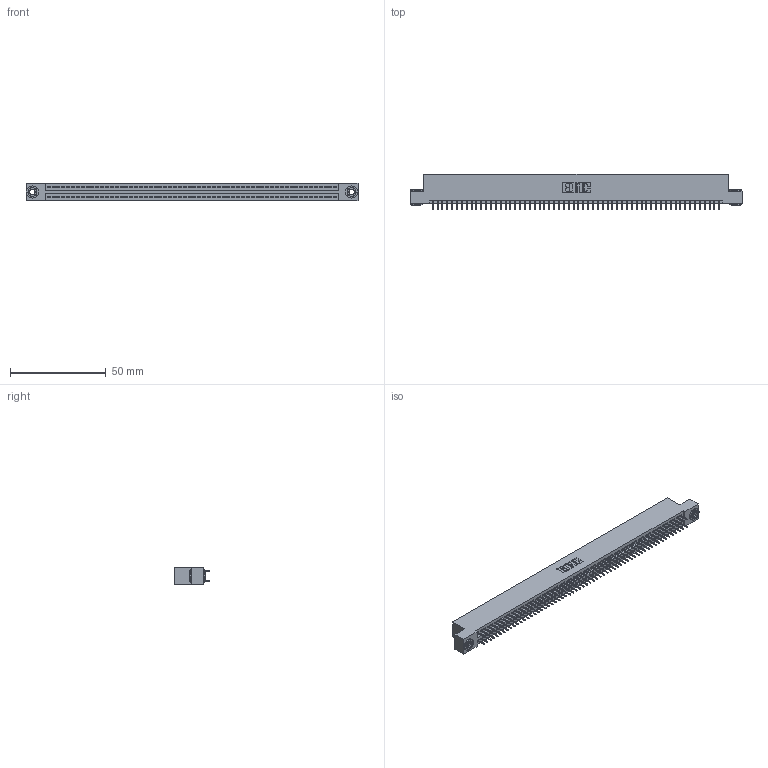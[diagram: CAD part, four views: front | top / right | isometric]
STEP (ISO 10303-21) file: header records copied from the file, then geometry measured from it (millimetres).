
FILE_DESCRIPTION (( 'STEP AP203' ), '1' );
FILE_NAME ('845-120-525-203.STEP', '2020-09-24T09:25:24', ( '' ), ( '' ), 'SwSTEP 2.0', 'SolidWorks 2020', '' );
FILE_SCHEMA (( 'CONFIG_CONTROL_DESIGN' ));
Length unit declared in the file: inch
Products named in the file (4): 345-250-002_345-250-002-102; 845-120-525-203; 345-292-001_345-293-125; 845 Part_Flush Mounting Lugs - 0.156 Dia-TH
Assembly tree (123 placements, depth 2):
  845-120-525-203
    845 Part_Flush Mounting Lugs - 0.156 Dia-TH
    345-292-001_345-293-125  x120
    345-250-002_345-250-002-102  x2
Bounding box: 173.61 x 18.72 x 9.4 mm (x, y, z)
Volume: 16853.5 mm3; surface area: 24870.6 mm2
Topology: 123 solids, 123 shells, 6644 faces, 18777 edges, 12034 vertices
Faces by surface type: plane 4770, cylinder 1866, cone 8
Entity records: 45378 total; most frequent: CARTESIAN_POINT 7563, ORIENTED_EDGE 7490, DIRECTION 6679, EDGE_CURVE 3745, VECTOR 3353, LINE 3353, VERTEX_POINT 2490, AXIS2_PLACEMENT_3D 1663
